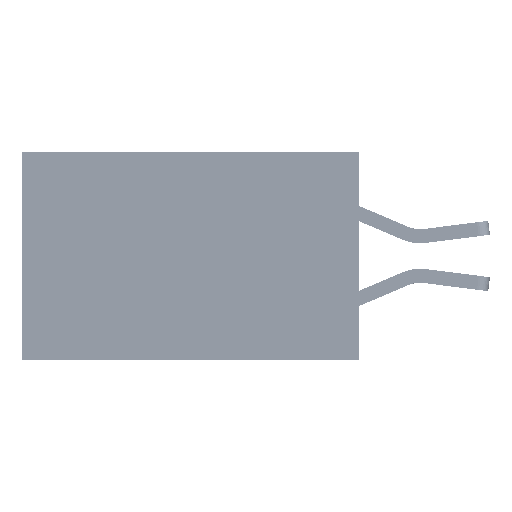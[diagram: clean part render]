
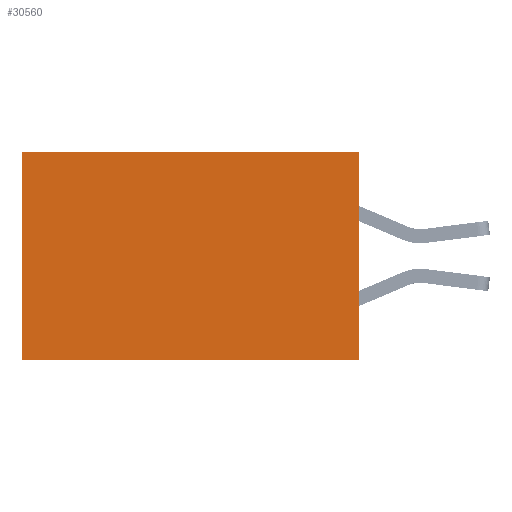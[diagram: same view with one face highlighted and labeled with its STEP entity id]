
A CAD part, left-side view. The second image highlights one B-rep face of the part: STEP entity #30560.
In plain terms, the highlighted planar face has unit normal (-1, 0, 0).
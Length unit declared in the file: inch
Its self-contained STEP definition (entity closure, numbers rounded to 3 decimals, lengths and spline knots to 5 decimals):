
#846 = DIRECTION ( 'NONE',  ( 0., 1., 0. ) ) ;
#1377 = CARTESIAN_POINT ( 'NONE',  ( 0.2875, 0., 0. ) ) ;
#4901 = LINE ( 'NONE', #48896, #10599 ) ;
#7236 = FACE_OUTER_BOUND ( 'NONE', #45214, .T. ) ;
#8340 = ORIENTED_EDGE ( 'NONE', *, *, #18859, .T. ) ;
#10599 = VECTOR ( 'NONE', #846, 39.37008 ) ;
#15143 = VECTOR ( 'NONE', #31361, 39.37008 ) ;
#15868 = EDGE_CURVE ( 'NONE', #18275, #16683, #4901, .T. ) ;
#16683 = VERTEX_POINT ( 'NONE', #18496 ) ;
#18275 = VERTEX_POINT ( 'NONE', #33544 ) ;
#18496 = CARTESIAN_POINT ( 'NONE',  ( 0.2875, 0.6, -0.37 ) ) ;
#18859 = EDGE_CURVE ( 'NONE', #25294, #16683, #19131, .T. ) ;
#19131 = LINE ( 'NONE', #36354, #52124 ) ;
#22545 = ORIENTED_EDGE ( 'NONE', *, *, #27342, .T. ) ;
#23268 = CARTESIAN_POINT ( 'NONE',  ( 0.2875, 0., 0. ) ) ;
#23612 = VERTEX_POINT ( 'NONE', #38392 ) ;
#24934 = DIRECTION ( 'NONE',  ( 1., 0., 0. ) ) ;
#25283 = DIRECTION ( 'NONE',  ( 0., 0., -1. ) ) ;
#25294 = VERTEX_POINT ( 'NONE', #26930 ) ;
#25892 = LINE ( 'NONE', #23268, #15143 ) ;
#26930 = CARTESIAN_POINT ( 'NONE',  ( 0.2875, 0.6, 0. ) ) ;
#27273 = EDGE_CURVE ( 'NONE', #23612, #18275, #28980, .T. ) ;
#27310 = DIRECTION ( 'NONE',  ( 0., 0., -1. ) ) ;
#27342 = EDGE_CURVE ( 'NONE', #23612, #25294, #25892, .T. ) ;
#28843 = DIRECTION ( 'NONE',  ( 0., 0., -1. ) ) ;
#28980 = LINE ( 'NONE', #40095, #37949 ) ;
#29417 = ORIENTED_EDGE ( 'NONE', *, *, #15868, .F. ) ;
#30560 = ADVANCED_FACE ( 'NONE', ( #7236 ), #37344, .F. ) ;
#31361 = DIRECTION ( 'NONE',  ( 0., 1., 0. ) ) ;
#33544 = CARTESIAN_POINT ( 'NONE',  ( 0.2875, 0., -0.37 ) ) ;
#34436 = ORIENTED_EDGE ( 'NONE', *, *, #27273, .F. ) ;
#36354 = CARTESIAN_POINT ( 'NONE',  ( 0.2875, 0.6, 0. ) ) ;
#37344 = PLANE ( 'NONE',  #43716 ) ;
#37949 = VECTOR ( 'NONE', #27310, 39.37008 ) ;
#38392 = CARTESIAN_POINT ( 'NONE',  ( 0.2875, 0., 0. ) ) ;
#40095 = CARTESIAN_POINT ( 'NONE',  ( 0.2875, 0., 0. ) ) ;
#43716 = AXIS2_PLACEMENT_3D ( 'NONE', #1377, #24934, #25283 ) ;
#45214 = EDGE_LOOP ( 'NONE', ( #8340, #29417, #34436, #22545 ) ) ;
#48896 = CARTESIAN_POINT ( 'NONE',  ( 0.2875, 0., -0.37 ) ) ;
#52124 = VECTOR ( 'NONE', #28843, 39.37008 ) ;
